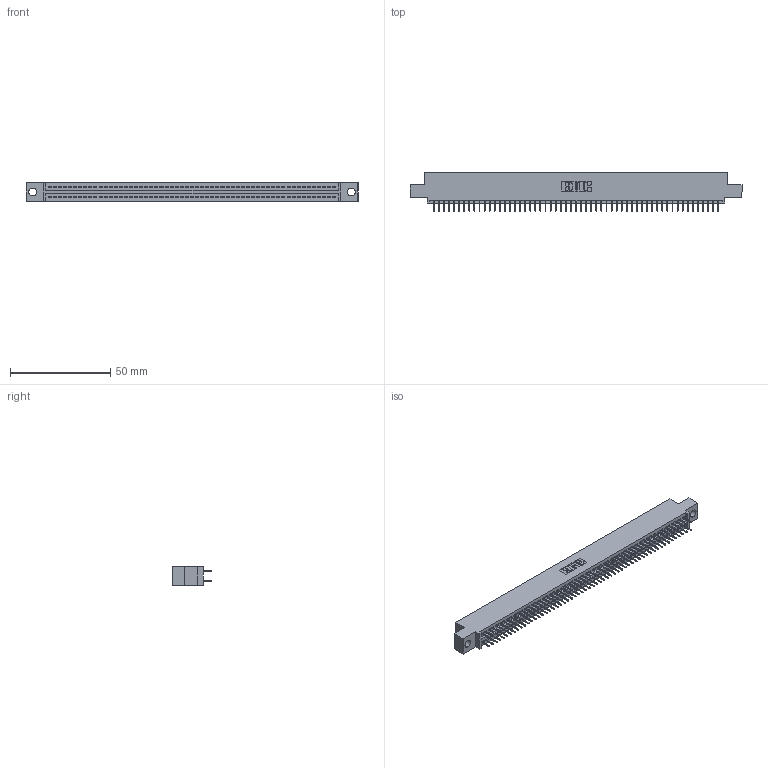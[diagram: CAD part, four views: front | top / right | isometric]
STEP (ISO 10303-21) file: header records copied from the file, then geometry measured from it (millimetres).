
FILE_DESCRIPTION (( 'STEP AP203' ), '1' );
FILE_NAME ('395-114-524-504.STEP', '2018-12-01T15:19:46', ( '' ), ( '' ), 'SwSTEP 2.0', 'SolidWorks 2016', '' );
FILE_SCHEMA (( 'CONFIG_CONTROL_DESIGN' ));
Length unit declared in the file: inch
Products named in the file (3): 345 Part_0.110 Offset - 0.156 Dia-TH; 395-114-524-504; 345-292-001_345-293-124
Assembly tree (115 placements, depth 2):
  395-114-524-504
    345 Part_0.110 Offset - 0.156 Dia-TH
    345-292-001_345-293-124  x114
Bounding box: 165.99 x 19.35 x 9.4 mm (x, y, z)
Volume: 15929.8 mm3; surface area: 23290.1 mm2
Topology: 115 solids, 115 shells, 6286 faces, 17795 edges, 11406 vertices
Faces by surface type: plane 4530, cylinder 1756
Entity records: 42913 total; most frequent: CARTESIAN_POINT 7180, ORIENTED_EDGE 7114, DIRECTION 6313, EDGE_CURVE 3557, VECTOR 3201, LINE 3201, VERTEX_POINT 2366, AXIS2_PLACEMENT_3D 1556
